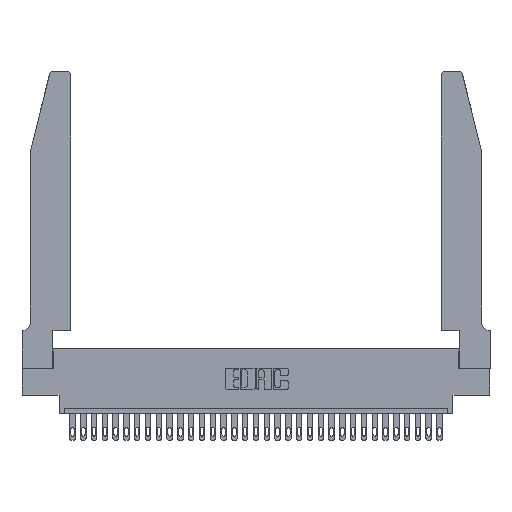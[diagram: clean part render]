
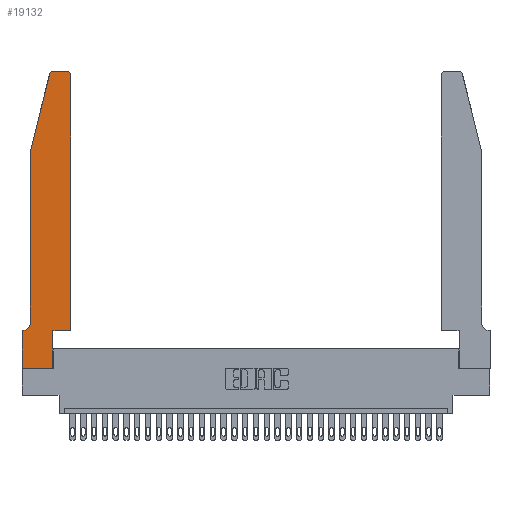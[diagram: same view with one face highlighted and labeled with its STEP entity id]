
A CAD part, top view. The second image highlights one B-rep face of the part: STEP entity #19132.
In plain terms, the highlighted planar face has unit normal (0, 0, 1).
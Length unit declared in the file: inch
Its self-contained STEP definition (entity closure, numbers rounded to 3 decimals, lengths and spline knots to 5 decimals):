
#328 = CARTESIAN_POINT ( 'NONE',  ( 0.0055, 0.42, 0.37 ) ) ;
#809 = ORIENTED_EDGE ( 'NONE', *, *, #12856, .T. ) ;
#944 = ORIENTED_EDGE ( 'NONE', *, *, #28533, .T. ) ;
#956 = CARTESIAN_POINT ( 'NONE',  ( 0.2865, 0., 0.37 ) ) ;
#1546 = CARTESIAN_POINT ( 'NONE',  ( 0.4505, 0.35, 0.37 ) ) ;
#1864 = CARTESIAN_POINT ( 'NONE',  ( 0.4505, 2.72, 0.37 ) ) ;
#2885 = EDGE_LOOP ( 'NONE', ( #14519, #809, #28284, #32126, #3695, #13493, #27305, #16900, #13705, #21193, #944, #4811 ) ) ;
#3064 = VERTEX_POINT ( 'NONE', #7760 ) ;
#3695 = ORIENTED_EDGE ( 'NONE', *, *, #23224, .T. ) ;
#3807 = CARTESIAN_POINT ( 'NONE',  ( 0., 0., 0.37 ) ) ;
#4226 = FACE_OUTER_BOUND ( 'NONE', #2885, .T. ) ;
#4265 = CARTESIAN_POINT ( 'NONE',  ( 0.284, 2.75, 0.37 ) ) ;
#4315 = AXIS2_PLACEMENT_3D ( 'NONE', #15199, #5442, #10113 ) ;
#4811 = ORIENTED_EDGE ( 'NONE', *, *, #16238, .T. ) ;
#4944 = LINE ( 'NONE', #26202, #14257 ) ;
#5442 = DIRECTION ( 'NONE',  ( 0., 0., 1. ) ) ;
#5794 = CARTESIAN_POINT ( 'NONE',  ( 0.0755, 0.35, 0.37 ) ) ;
#5972 = EDGE_CURVE ( 'NONE', #25303, #18222, #4944, .T. ) ;
#7034 = CIRCLE ( 'NONE', #8969, 0.03 ) ;
#7157 = EDGE_CURVE ( 'NONE', #11411, #18852, #7180, .T. ) ;
#7180 = LINE ( 'NONE', #28428, #22296 ) ;
#7285 = VECTOR ( 'NONE', #17344, 39.37008 ) ;
#7760 = CARTESIAN_POINT ( 'NONE',  ( 0.4205, 2.75, 0.37 ) ) ;
#8726 = AXIS2_PLACEMENT_3D ( 'NONE', #328, #15456, #22502 ) ;
#8927 = CARTESIAN_POINT ( 'NONE',  ( 0., 0., 0.37 ) ) ;
#8969 = AXIS2_PLACEMENT_3D ( 'NONE', #28050, #17446, #10168 ) ;
#9144 = DIRECTION ( 'NONE',  ( 0., 0., 1. ) ) ;
#9282 = VECTOR ( 'NONE', #11820, 39.37008 ) ;
#9373 = VERTEX_POINT ( 'NONE', #13803 ) ;
#9873 = DIRECTION ( 'NONE',  ( 1., 0., 0. ) ) ;
#10113 = DIRECTION ( 'NONE',  ( 1., 0., 0. ) ) ;
#10168 = DIRECTION ( 'NONE',  ( 1., 0., 0. ) ) ;
#10216 = PLANE ( 'NONE',  #4315 ) ;
#10357 = VERTEX_POINT ( 'NONE', #1864 ) ;
#10831 = LINE ( 'NONE', #26688, #9282 ) ;
#11105 = AXIS2_PLACEMENT_3D ( 'NONE', #23987, #9144, #26510 ) ;
#11411 = VERTEX_POINT ( 'NONE', #31953 ) ;
#11739 = DIRECTION ( 'NONE',  ( -1., 0., 0. ) ) ;
#11820 = DIRECTION ( 'NONE',  ( 0., 1., 0. ) ) ;
#12234 = VECTOR ( 'NONE', #12889, 39.37008 ) ;
#12856 = EDGE_CURVE ( 'NONE', #25574, #21218, #7034, .T. ) ;
#12889 = DIRECTION ( 'NONE',  ( -0.239, -0.971, 0. ) ) ;
#13057 = DIRECTION ( 'NONE',  ( -1., 0., 0. ) ) ;
#13493 = ORIENTED_EDGE ( 'NONE', *, *, #23349, .T. ) ;
#13538 = CARTESIAN_POINT ( 'NONE',  ( 0.0055, 0.35, 0.37 ) ) ;
#13576 = DIRECTION ( 'NONE',  ( 0., -1., 0. ) ) ;
#13705 = ORIENTED_EDGE ( 'NONE', *, *, #5972, .T. ) ;
#13803 = CARTESIAN_POINT ( 'NONE',  ( 0.0755, 2., 0.37 ) ) ;
#13816 = EDGE_CURVE ( 'NONE', #18852, #25303, #15922, .T. ) ;
#14257 = VECTOR ( 'NONE', #25887, 39.37008 ) ;
#14318 = LINE ( 'NONE', #5794, #22085 ) ;
#14519 = ORIENTED_EDGE ( 'NONE', *, *, #22025, .T. ) ;
#14666 = LINE ( 'NONE', #27203, #7285 ) ;
#15199 = CARTESIAN_POINT ( 'NONE',  ( 0., 0.35, 0.37 ) ) ;
#15456 = DIRECTION ( 'NONE',  ( 0., 0., -1. ) ) ;
#15922 = LINE ( 'NONE', #8927, #27572 ) ;
#16238 = EDGE_CURVE ( 'NONE', #10357, #3064, #24608, .T. ) ;
#16900 = ORIENTED_EDGE ( 'NONE', *, *, #13816, .T. ) ;
#16922 = EDGE_CURVE ( 'NONE', #18222, #24853, #24576, .T. ) ;
#17344 = DIRECTION ( 'NONE',  ( 0., -1., 0. ) ) ;
#17446 = DIRECTION ( 'NONE',  ( 0., 0., 1. ) ) ;
#18222 = VERTEX_POINT ( 'NONE', #22476 ) ;
#18852 = VERTEX_POINT ( 'NONE', #3807 ) ;
#19132 = ADVANCED_FACE ( 'NONE', ( #4226 ), #10216, .T. ) ;
#19266 = CARTESIAN_POINT ( 'NONE',  ( 0.0755, 0.42, 0.37 ) ) ;
#19619 = LINE ( 'NONE', #20284, #12234 ) ;
#20253 = VERTEX_POINT ( 'NONE', #19266 ) ;
#20284 = CARTESIAN_POINT ( 'NONE',  ( 0.0755, 2., 0.37 ) ) ;
#21193 = ORIENTED_EDGE ( 'NONE', *, *, #16922, .T. ) ;
#21218 = VERTEX_POINT ( 'NONE', #26761 ) ;
#21294 = CIRCLE ( 'NONE', #8726, 0.07 ) ;
#21763 = VECTOR ( 'NONE', #11739, 39.37008 ) ;
#21806 = CARTESIAN_POINT ( 'NONE',  ( 0.2605, 2.75, 0.37 ) ) ;
#22025 = EDGE_CURVE ( 'NONE', #3064, #25574, #26826, .T. ) ;
#22085 = VECTOR ( 'NONE', #13057, 39.37008 ) ;
#22296 = VECTOR ( 'NONE', #13576, 39.37008 ) ;
#22336 = CARTESIAN_POINT ( 'NONE',  ( 0.4505, 0.35, 0.37 ) ) ;
#22476 = CARTESIAN_POINT ( 'NONE',  ( 0.2865, 0.35, 0.37 ) ) ;
#22502 = DIRECTION ( 'NONE',  ( -1., 0., 0. ) ) ;
#23224 = EDGE_CURVE ( 'NONE', #20253, #26669, #21294, .T. ) ;
#23349 = EDGE_CURVE ( 'NONE', #26669, #11411, #14318, .T. ) ;
#23787 = VECTOR ( 'NONE', #9873, 39.37008 ) ;
#23987 = CARTESIAN_POINT ( 'NONE',  ( 0.4205, 2.72, 0.37 ) ) ;
#24576 = LINE ( 'NONE', #22336, #23787 ) ;
#24608 = CIRCLE ( 'NONE', #11105, 0.03 ) ;
#24853 = VERTEX_POINT ( 'NONE', #1546 ) ;
#25303 = VERTEX_POINT ( 'NONE', #956 ) ;
#25574 = VERTEX_POINT ( 'NONE', #4265 ) ;
#25887 = DIRECTION ( 'NONE',  ( 0., 1., 0. ) ) ;
#26202 = CARTESIAN_POINT ( 'NONE',  ( 0.2865, 0.35, 0.37 ) ) ;
#26510 = DIRECTION ( 'NONE',  ( 1., 0., 0. ) ) ;
#26669 = VERTEX_POINT ( 'NONE', #13538 ) ;
#26688 = CARTESIAN_POINT ( 'NONE',  ( 0.4505, 0.35, 0.37 ) ) ;
#26761 = CARTESIAN_POINT ( 'NONE',  ( 0.25487, 2.72718, 0.37 ) ) ;
#26826 = LINE ( 'NONE', #21806, #21763 ) ;
#27203 = CARTESIAN_POINT ( 'NONE',  ( 0.0755, 2., 0.37 ) ) ;
#27305 = ORIENTED_EDGE ( 'NONE', *, *, #7157, .T. ) ;
#27572 = VECTOR ( 'NONE', #30954, 39.37008 ) ;
#28050 = CARTESIAN_POINT ( 'NONE',  ( 0.284, 2.72, 0.37 ) ) ;
#28284 = ORIENTED_EDGE ( 'NONE', *, *, #31154, .T. ) ;
#28428 = CARTESIAN_POINT ( 'NONE',  ( 0., 0., 0.37 ) ) ;
#28533 = EDGE_CURVE ( 'NONE', #24853, #10357, #10831, .T. ) ;
#29777 = EDGE_CURVE ( 'NONE', #9373, #20253, #14666, .T. ) ;
#30954 = DIRECTION ( 'NONE',  ( 1., 0., 0. ) ) ;
#31154 = EDGE_CURVE ( 'NONE', #21218, #9373, #19619, .T. ) ;
#31953 = CARTESIAN_POINT ( 'NONE',  ( 0., 0.35, 0.37 ) ) ;
#32126 = ORIENTED_EDGE ( 'NONE', *, *, #29777, .T. ) ;
